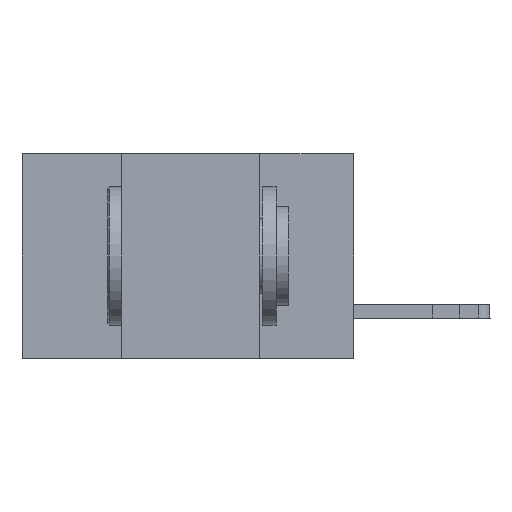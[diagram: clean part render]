
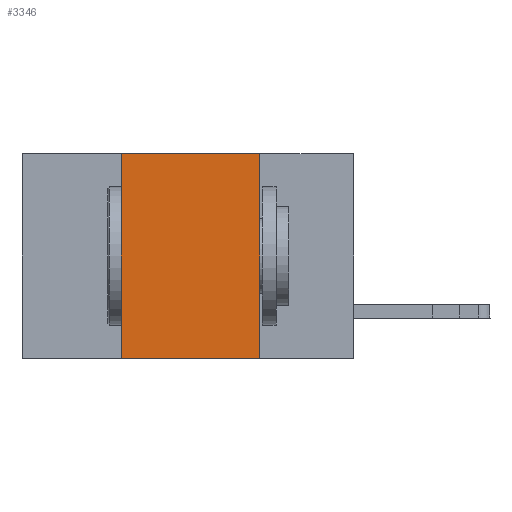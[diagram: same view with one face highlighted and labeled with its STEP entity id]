
A CAD part, left-side view. The second image highlights one B-rep face of the part: STEP entity #3346.
In plain terms, the highlighted planar face has unit normal (-1, 0, 0).
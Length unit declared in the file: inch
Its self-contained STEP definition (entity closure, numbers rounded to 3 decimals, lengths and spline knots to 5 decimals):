
#136 = CARTESIAN_POINT ( 'NONE',  ( 0., 0.17, -0.37 ) ) ;
#1168 = CARTESIAN_POINT ( 'NONE',  ( 0., 0.42, -0.37 ) ) ;
#1372 = VECTOR ( 'NONE', #4377, 39.37008 ) ;
#2265 = EDGE_CURVE ( 'NONE', #2908, #3764, #5966, .T. ) ;
#2908 = VERTEX_POINT ( 'NONE', #22216 ) ;
#3346 = ADVANCED_FACE ( 'NONE', ( #24805 ), #20517, .F. ) ;
#3761 = EDGE_CURVE ( 'NONE', #14340, #18293, #19799, .T. ) ;
#3764 = VERTEX_POINT ( 'NONE', #136 ) ;
#4013 = AXIS2_PLACEMENT_3D ( 'NONE', #10925, #16950, #24415 ) ;
#4377 = DIRECTION ( 'NONE',  ( 0., -1., 0. ) ) ;
#5573 = DIRECTION ( 'NONE',  ( 0., -1., 0. ) ) ;
#5854 = DIRECTION ( 'NONE',  ( 0., 0., -1. ) ) ;
#5966 = LINE ( 'NONE', #23157, #24344 ) ;
#6966 = ORIENTED_EDGE ( 'NONE', *, *, #3761, .F. ) ;
#10925 = CARTESIAN_POINT ( 'NONE',  ( 0., 0.6, 0. ) ) ;
#11214 = VECTOR ( 'NONE', #5573, 39.37008 ) ;
#12856 = VECTOR ( 'NONE', #13974, 39.37008 ) ;
#13974 = DIRECTION ( 'NONE',  ( 0., 0., 1. ) ) ;
#14340 = VERTEX_POINT ( 'NONE', #1168 ) ;
#14369 = EDGE_CURVE ( 'NONE', #14340, #3764, #20597, .T. ) ;
#15451 = CARTESIAN_POINT ( 'NONE',  ( 0., 0.6, 0. ) ) ;
#16950 = DIRECTION ( 'NONE',  ( 1., 0., 0. ) ) ;
#17719 = ORIENTED_EDGE ( 'NONE', *, *, #14369, .T. ) ;
#18293 = VERTEX_POINT ( 'NONE', #21000 ) ;
#18688 = CARTESIAN_POINT ( 'NONE',  ( 0., 0.6, -0.37 ) ) ;
#19336 = ORIENTED_EDGE ( 'NONE', *, *, #2265, .F. ) ;
#19522 = LINE ( 'NONE', #15451, #1372 ) ;
#19674 = CARTESIAN_POINT ( 'NONE',  ( 0., 0.42, 0. ) ) ;
#19799 = LINE ( 'NONE', #19674, #12856 ) ;
#20517 = PLANE ( 'NONE',  #4013 ) ;
#20597 = LINE ( 'NONE', #18688, #11214 ) ;
#21000 = CARTESIAN_POINT ( 'NONE',  ( 0., 0.42, 0. ) ) ;
#21149 = ORIENTED_EDGE ( 'NONE', *, *, #23217, .F. ) ;
#22216 = CARTESIAN_POINT ( 'NONE',  ( 0., 0.17, 0. ) ) ;
#23157 = CARTESIAN_POINT ( 'NONE',  ( 0., 0.17, 0. ) ) ;
#23217 = EDGE_CURVE ( 'NONE', #18293, #2908, #19522, .T. ) ;
#23656 = EDGE_LOOP ( 'NONE', ( #19336, #21149, #6966, #17719 ) ) ;
#24344 = VECTOR ( 'NONE', #5854, 39.37008 ) ;
#24415 = DIRECTION ( 'NONE',  ( 0., 0., -1. ) ) ;
#24805 = FACE_OUTER_BOUND ( 'NONE', #23656, .T. ) ;
